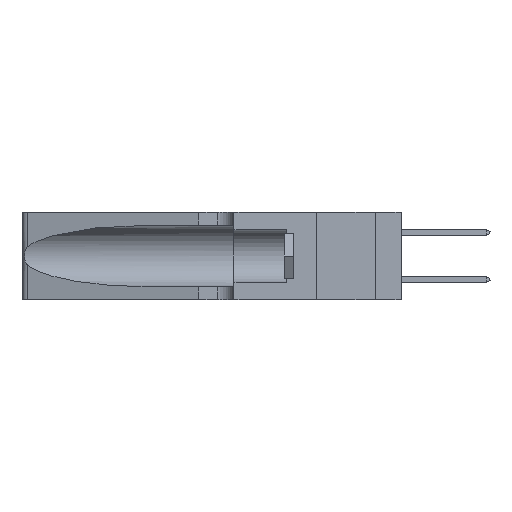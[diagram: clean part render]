
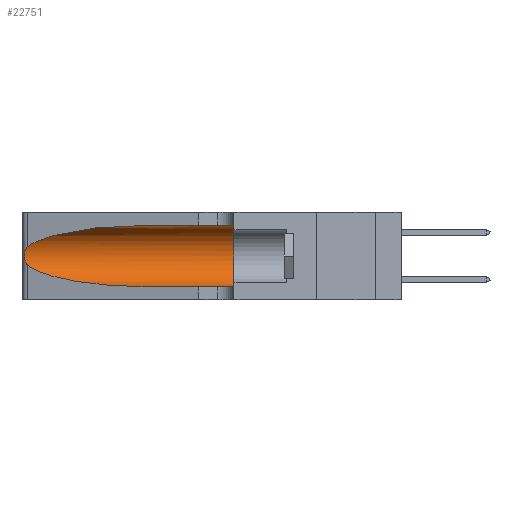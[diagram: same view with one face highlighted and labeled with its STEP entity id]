
A CAD part, left-side view. The second image highlights one B-rep face of the part: STEP entity #22751.
In plain terms, the highlighted cylindrical face has radius 3.308 mm (diameter 6.617 mm), a partial arc.
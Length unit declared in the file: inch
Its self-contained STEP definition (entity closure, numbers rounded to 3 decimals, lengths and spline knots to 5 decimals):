
#558 = CARTESIAN_POINT ( 'NONE',  ( 0.1305, 0.35, 0.05475 ) ) ;
#634 = CARTESIAN_POINT ( 'NONE',  ( 0.25487, 1.22718, 0.14631 ) ) ;
#846 = CIRCLE ( 'NONE', #15056, 0.13025 ) ;
#1341 = CARTESIAN_POINT ( 'NONE',  ( 0.1305, 0.35, 0.185 ) ) ;
#2648 = VERTEX_POINT ( 'NONE', #8470 ) ;
#2679 = CARTESIAN_POINT ( 'NONE',  ( 0.25639, 1.23184, 0.21858 ) ) ;
#2754 = VERTEX_POINT ( 'NONE', #23849 ) ;
#2785 = DIRECTION ( 'NONE',  ( 0., -1., 0. ) ) ;
#3995 = ORIENTED_EDGE ( 'NONE', *, *, #7959, .T. ) ;
#4475 = CARTESIAN_POINT ( 'NONE',  ( 0.25856, 1.23593, 0.16098 ) ) ;
#5218 = CARTESIAN_POINT ( 'NONE',  ( 0.1305, 1.61858, 0.185 ) ) ;
#5350 = EDGE_CURVE ( 'NONE', #2648, #12804, #846, .T. ) ;
#5849 = AXIS2_PLACEMENT_3D ( 'NONE', #5218, #16584, #14716 ) ;
#6271 = CARTESIAN_POINT ( 'NONE',  ( 0.26018, 1.23835, 0.19895 ) ) ;
#6541 = ORIENTED_EDGE ( 'NONE', *, *, #13703, .F. ) ;
#6627 = CARTESIAN_POINT ( 'NONE',  ( 0.1305, 1.61858, 0.05475 ) ) ;
#7047 = CARTESIAN_POINT ( 'NONE',  ( 0.2373, 1.15595, 0.08982 ) ) ;
#7624 = CARTESIAN_POINT ( 'NONE',  ( 0.25487, 1.22718, 0.22369 ) ) ;
#7959 = EDGE_CURVE ( 'NONE', #2754, #14787, #15832, .T. ) ;
#8470 = CARTESIAN_POINT ( 'NONE',  ( 0.1305, 0.35, 0.31525 ) ) ;
#8500 = ORIENTED_EDGE ( 'NONE', *, *, #5350, .F. ) ;
#8917 = VECTOR ( 'NONE', #2785, 39.37008 ) ;
#9363 = CARTESIAN_POINT ( 'NONE',  ( 0.25487, 1.22718, 0.22369 ) ) ;
#9440 = CYLINDRICAL_SURFACE ( 'NONE', #5849, 0.13025 ) ;
#9722 = VERTEX_POINT ( 'NONE', #23989 ) ;
#9944 = CARTESIAN_POINT ( 'NONE',  ( 0.25639, 1.23186, 0.15144 ) ) ;
#10052 = ORIENTED_EDGE ( 'NONE', *, *, #17710, .T. ) ;
#10483 = CARTESIAN_POINT ( 'NONE',  ( 0.18966, 0.96281, 0.05475 ) ) ;
#11825 = CARTESIAN_POINT ( 'NONE',  ( 0.25555, 1.22993, 0.14849 ) ) ;
#12804 = VERTEX_POINT ( 'NONE', #558 ) ;
#13703 = EDGE_CURVE ( 'NONE', #2754, #2648, #15787, .T. ) ;
#13726 = CARTESIAN_POINT ( 'NONE',  ( 0.1305, 1.61858, 0.31525 ) ) ;
#13760 = VECTOR ( 'NONE', #21254, 39.37008 ) ;
#13818 = VERTEX_POINT ( 'NONE', #17894 ) ;
#14015 =( BOUNDED_CURVE ( )  B_SPLINE_CURVE ( 3, ( #14491, #7047, #10483, #18158 ),
 .UNSPECIFIED., .F., .F. ) 
 B_SPLINE_CURVE_WITH_KNOTS ( ( 4, 4 ),
 ( 3.44316, 4.71239 ),
 .UNSPECIFIED. ) 
 CURVE ( )  GEOMETRIC_REPRESENTATION_ITEM ( )  RATIONAL_B_SPLINE_CURVE ( ( 1., 0.87, 0.87, 1. ) ) 
 REPRESENTATION_ITEM ( '' )  );
#14033 = CARTESIAN_POINT ( 'NONE',  ( 0.25854, 1.2359, 0.20912 ) ) ;
#14491 = CARTESIAN_POINT ( 'NONE',  ( 0.25487, 1.22718, 0.14631 ) ) ;
#14553 = CARTESIAN_POINT ( 'NONE',  ( 0.18966, 0.96281, 0.31525 ) ) ;
#14716 = DIRECTION ( 'NONE',  ( 0., 0., -1. ) ) ;
#14787 = VERTEX_POINT ( 'NONE', #7624 ) ;
#15020 = FACE_OUTER_BOUND ( 'NONE', #15659, .T. ) ;
#15056 = AXIS2_PLACEMENT_3D ( 'NONE', #1341, #18319, #21849 ) ;
#15659 = EDGE_LOOP ( 'NONE', ( #3995, #23674, #23573, #10052, #8500, #6541 ) ) ;
#15787 = LINE ( 'NONE', #13726, #13760 ) ;
#15832 =( BOUNDED_CURVE ( )  B_SPLINE_CURVE ( 3, ( #20655, #14553, #21175, #9363 ),
 .UNSPECIFIED., .F., .F. ) 
 B_SPLINE_CURVE_WITH_KNOTS ( ( 4, 4 ),
 ( 1.5708, 2.84003 ),
 .UNSPECIFIED. ) 
 CURVE ( )  GEOMETRIC_REPRESENTATION_ITEM ( )  RATIONAL_B_SPLINE_CURVE ( ( 1., 0.87, 0.87, 1. ) ) 
 REPRESENTATION_ITEM ( '' )  );
#15839 = CARTESIAN_POINT ( 'NONE',  ( 0.26017, 1.23833, 0.17102 ) ) ;
#16584 = DIRECTION ( 'NONE',  ( 0., -1., 0. ) ) ;
#17468 = CARTESIAN_POINT ( 'NONE',  ( 0.25787, 1.23484, 0.2124 ) ) ;
#17709 = CARTESIAN_POINT ( 'NONE',  ( 0.26075, 1.23896, 0.19203 ) ) ;
#17710 = EDGE_CURVE ( 'NONE', #13818, #12804, #22673, .T. ) ;
#17796 = CARTESIAN_POINT ( 'NONE',  ( 0.25487, 1.22718, 0.22369 ) ) ;
#17894 = CARTESIAN_POINT ( 'NONE',  ( 0.1305, 0.72297, 0.05475 ) ) ;
#18158 = CARTESIAN_POINT ( 'NONE',  ( 0.1305, 0.72297, 0.05475 ) ) ;
#18169 = EDGE_CURVE ( 'NONE', #14787, #9722, #23797, .T. ) ;
#18319 = DIRECTION ( 'NONE',  ( 0., 1., 0. ) ) ;
#19028 = EDGE_CURVE ( 'NONE', #9722, #13818, #14015, .T. ) ;
#19432 = CARTESIAN_POINT ( 'NONE',  ( 0.25555, 1.22994, 0.2215 ) ) ;
#20655 = CARTESIAN_POINT ( 'NONE',  ( 0.1305, 0.72297, 0.31525 ) ) ;
#21175 = CARTESIAN_POINT ( 'NONE',  ( 0.2373, 1.15595, 0.28018 ) ) ;
#21254 = DIRECTION ( 'NONE',  ( 0., -1., 0. ) ) ;
#21849 = DIRECTION ( 'NONE',  ( 0., 0., 1. ) ) ;
#22673 = LINE ( 'NONE', #6627, #8917 ) ;
#22751 = ADVANCED_FACE ( 'NONE', ( #15020 ), #9440, .F. ) ;
#23295 = CARTESIAN_POINT ( 'NONE',  ( 0.25789, 1.23486, 0.15765 ) ) ;
#23377 = CARTESIAN_POINT ( 'NONE',  ( 0.26075, 1.23896, 0.178 ) ) ;
#23573 = ORIENTED_EDGE ( 'NONE', *, *, #19028, .T. ) ;
#23674 = ORIENTED_EDGE ( 'NONE', *, *, #18169, .T. ) ;
#23797 = B_SPLINE_CURVE_WITH_KNOTS ( 'NONE', 3,
 ( #17796, #19432, #2679, #17468, #14033, #6271, #17709, #23377, #15839, #4475, #23295, #9944, #11825, #634 ),
 .UNSPECIFIED., .F., .F.,
 ( 4, 2, 2, 2, 2, 2, 4 ),
 ( 0., 0.00027, 0.00053, 0.00107, 0.0016, 0.00187, 0.00214 ),
 .UNSPECIFIED. ) ;
#23849 = CARTESIAN_POINT ( 'NONE',  ( 0.1305, 0.72297, 0.31525 ) ) ;
#23989 = CARTESIAN_POINT ( 'NONE',  ( 0.25487, 1.22718, 0.14631 ) ) ;
